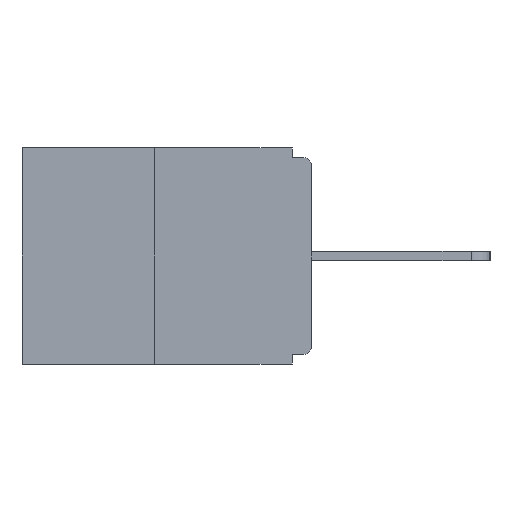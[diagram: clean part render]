
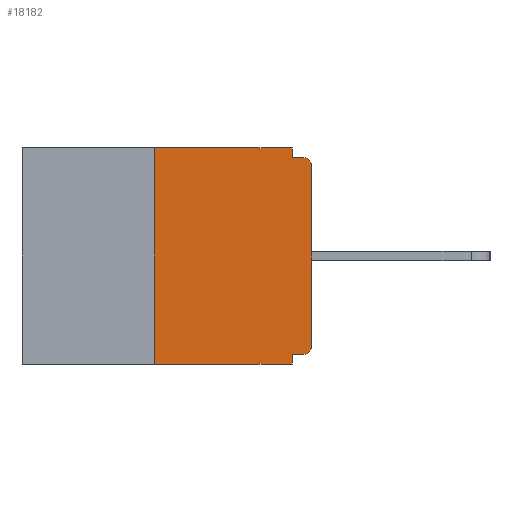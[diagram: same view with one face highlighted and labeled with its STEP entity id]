
A CAD part, left-side view. The second image highlights one B-rep face of the part: STEP entity #18182.
In plain terms, the highlighted planar face has unit normal (-1, 0, 0).
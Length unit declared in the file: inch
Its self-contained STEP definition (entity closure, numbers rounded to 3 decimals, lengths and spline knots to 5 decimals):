
#62 = DIRECTION ( 'NONE',  ( -1., 0., 0. ) ) ;
#240 = LINE ( 'NONE', #15771, #6008 ) ;
#432 = EDGE_CURVE ( 'NONE', #2027, #8841, #4977, .T. ) ;
#460 = VERTEX_POINT ( 'NONE', #10391 ) ;
#983 = DIRECTION ( 'NONE',  ( 0., 0., 1. ) ) ;
#1126 = DIRECTION ( 'NONE',  ( 0., 0., -1. ) ) ;
#1340 = AXIS2_PLACEMENT_3D ( 'NONE', #11129, #13989, #1126 ) ;
#1455 = VECTOR ( 'NONE', #12552, 39.37008 ) ;
#1485 = DIRECTION ( 'NONE',  ( 0., 0., -1. ) ) ;
#1491 = VECTOR ( 'NONE', #17908, 39.37008 ) ;
#1722 = ORIENTED_EDGE ( 'NONE', *, *, #4901, .F. ) ;
#2027 = VERTEX_POINT ( 'NONE', #16216 ) ;
#2303 = VECTOR ( 'NONE', #16602, 39.37008 ) ;
#2328 = VERTEX_POINT ( 'NONE', #3045 ) ;
#2932 = EDGE_CURVE ( 'NONE', #8841, #4367, #240, .T. ) ;
#3045 = CARTESIAN_POINT ( 'NONE',  ( 0., 0.015, -0.328 ) ) ;
#3063 = LINE ( 'NONE', #10860, #15597 ) ;
#3271 = VERTEX_POINT ( 'NONE', #11103 ) ;
#3292 = DIRECTION ( 'NONE',  ( 0., 0., -1. ) ) ;
#3408 = CARTESIAN_POINT ( 'NONE',  ( 0., 0., -0.313 ) ) ;
#3475 = VERTEX_POINT ( 'NONE', #3408 ) ;
#3613 = EDGE_CURVE ( 'NONE', #2328, #460, #3063, .T. ) ;
#3685 = ORIENTED_EDGE ( 'NONE', *, *, #11895, .F. ) ;
#3692 = ORIENTED_EDGE ( 'NONE', *, *, #8530, .T. ) ;
#3871 = CIRCLE ( 'NONE', #9556, 0.015 ) ;
#4302 = DIRECTION ( 'NONE',  ( 0., -1., 0. ) ) ;
#4334 = ORIENTED_EDGE ( 'NONE', *, *, #10689, .F. ) ;
#4367 = VERTEX_POINT ( 'NONE', #9156 ) ;
#4612 = VERTEX_POINT ( 'NONE', #8565 ) ;
#4901 = EDGE_CURVE ( 'NONE', #460, #12312, #15085, .T. ) ;
#4977 = LINE ( 'NONE', #10562, #11232 ) ;
#5124 = CARTESIAN_POINT ( 'NONE',  ( 0., 0.25, 0. ) ) ;
#5511 = EDGE_CURVE ( 'NONE', #3475, #8396, #8325, .T. ) ;
#5752 = CIRCLE ( 'NONE', #6399, 0.015 ) ;
#6008 = VECTOR ( 'NONE', #4302, 39.37008 ) ;
#6399 = AXIS2_PLACEMENT_3D ( 'NONE', #17125, #62, #1485 ) ;
#6714 = CARTESIAN_POINT ( 'NONE',  ( 0., 0.015, -0.03 ) ) ;
#7149 = VECTOR ( 'NONE', #12250, 39.37008 ) ;
#7448 = VECTOR ( 'NONE', #983, 39.37008 ) ;
#7892 = FACE_OUTER_BOUND ( 'NONE', #15488, .T. ) ;
#8137 = DIRECTION ( 'NONE',  ( 0., 0., -1. ) ) ;
#8231 = CARTESIAN_POINT ( 'NONE',  ( 0., 0., 0. ) ) ;
#8325 = LINE ( 'NONE', #8231, #2303 ) ;
#8396 = VERTEX_POINT ( 'NONE', #13926 ) ;
#8397 = CARTESIAN_POINT ( 'NONE',  ( 0., 0.031, -0.343 ) ) ;
#8530 = EDGE_CURVE ( 'NONE', #3271, #12312, #8932, .T. ) ;
#8565 = CARTESIAN_POINT ( 'NONE',  ( 0., 0.25, 0. ) ) ;
#8841 = VERTEX_POINT ( 'NONE', #11329 ) ;
#8932 = LINE ( 'NONE', #17781, #7149 ) ;
#9156 = CARTESIAN_POINT ( 'NONE',  ( 0., 0.015, -0.015 ) ) ;
#9556 = AXIS2_PLACEMENT_3D ( 'NONE', #6714, #16876, #8137 ) ;
#10224 = ORIENTED_EDGE ( 'NONE', *, *, #10227, .T. ) ;
#10227 = EDGE_CURVE ( 'NONE', #2328, #3475, #5752, .T. ) ;
#10391 = CARTESIAN_POINT ( 'NONE',  ( 0., 0.031, -0.328 ) ) ;
#10532 = CARTESIAN_POINT ( 'NONE',  ( 0., 0.46, 0. ) ) ;
#10562 = CARTESIAN_POINT ( 'NONE',  ( 0., 0.031, 0. ) ) ;
#10689 = EDGE_CURVE ( 'NONE', #4612, #2027, #17548, .T. ) ;
#10860 = CARTESIAN_POINT ( 'NONE',  ( 0., 0., -0.328 ) ) ;
#11103 = CARTESIAN_POINT ( 'NONE',  ( 0., 0.25, -0.343 ) ) ;
#11129 = CARTESIAN_POINT ( 'NONE',  ( 0., 0.46, 0. ) ) ;
#11232 = VECTOR ( 'NONE', #3292, 39.37008 ) ;
#11329 = CARTESIAN_POINT ( 'NONE',  ( 0., 0.031, -0.015 ) ) ;
#11521 = ORIENTED_EDGE ( 'NONE', *, *, #3613, .F. ) ;
#11895 = EDGE_CURVE ( 'NONE', #3271, #4612, #17932, .T. ) ;
#11966 = ORIENTED_EDGE ( 'NONE', *, *, #432, .F. ) ;
#12250 = DIRECTION ( 'NONE',  ( 0., -1., 0. ) ) ;
#12312 = VERTEX_POINT ( 'NONE', #8397 ) ;
#12552 = DIRECTION ( 'NONE',  ( 0., 0., -1. ) ) ;
#13710 = DIRECTION ( 'NONE',  ( 0., 1., 0. ) ) ;
#13926 = CARTESIAN_POINT ( 'NONE',  ( 0., 0., -0.03 ) ) ;
#13989 = DIRECTION ( 'NONE',  ( 1., 0., 0. ) ) ;
#14055 = PLANE ( 'NONE',  #1340 ) ;
#15085 = LINE ( 'NONE', #16668, #1455 ) ;
#15446 = ORIENTED_EDGE ( 'NONE', *, *, #2932, .F. ) ;
#15488 = EDGE_LOOP ( 'NONE', ( #4334, #3685, #3692, #1722, #11521, #10224, #18011, #15581, #15446, #11966 ) ) ;
#15581 = ORIENTED_EDGE ( 'NONE', *, *, #18162, .T. ) ;
#15597 = VECTOR ( 'NONE', #13710, 39.37008 ) ;
#15771 = CARTESIAN_POINT ( 'NONE',  ( 0., 0., -0.015 ) ) ;
#16216 = CARTESIAN_POINT ( 'NONE',  ( 0., 0.031, 0. ) ) ;
#16602 = DIRECTION ( 'NONE',  ( 0., 0., 1. ) ) ;
#16668 = CARTESIAN_POINT ( 'NONE',  ( 0., 0.031, -0.343 ) ) ;
#16876 = DIRECTION ( 'NONE',  ( -1., 0., 0. ) ) ;
#17125 = CARTESIAN_POINT ( 'NONE',  ( 0., 0.015, -0.313 ) ) ;
#17548 = LINE ( 'NONE', #10532, #1491 ) ;
#17781 = CARTESIAN_POINT ( 'NONE',  ( 0., 0.46, -0.343 ) ) ;
#17908 = DIRECTION ( 'NONE',  ( 0., -1., 0. ) ) ;
#17932 = LINE ( 'NONE', #5124, #7448 ) ;
#18011 = ORIENTED_EDGE ( 'NONE', *, *, #5511, .T. ) ;
#18162 = EDGE_CURVE ( 'NONE', #8396, #4367, #3871, .T. ) ;
#18182 = ADVANCED_FACE ( 'NONE', ( #7892 ), #14055, .F. ) ;
